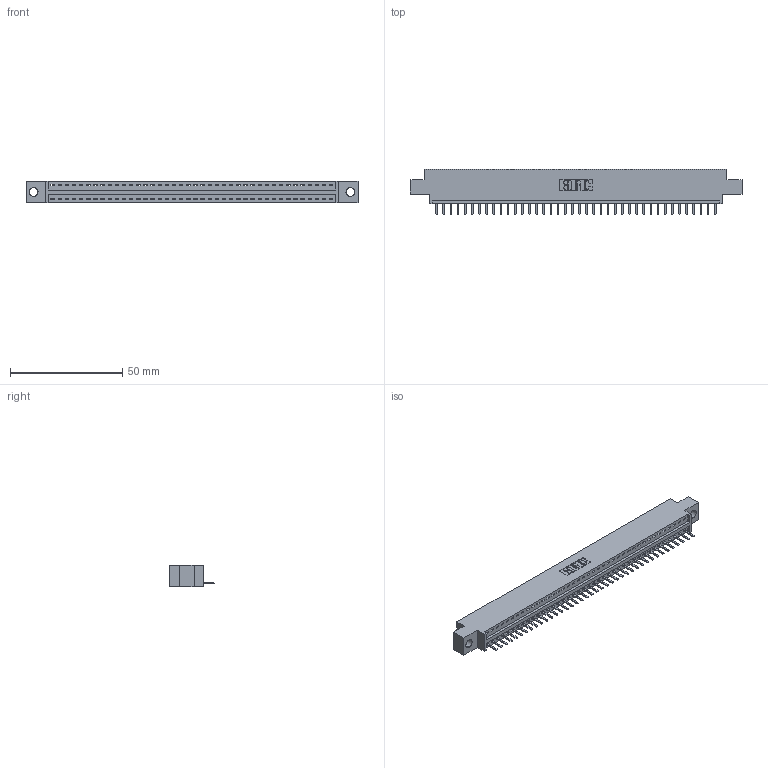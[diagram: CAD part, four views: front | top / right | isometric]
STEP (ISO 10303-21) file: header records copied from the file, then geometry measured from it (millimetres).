
FILE_DESCRIPTION (( 'STEP AP203' ), '1' );
FILE_NAME ('396-040-520-604.STEP', '2018-09-06T11:15:59', ( '' ), ( '' ), 'SwSTEP 2.0', 'SolidWorks 2016', '' );
FILE_SCHEMA (( 'CONFIG_CONTROL_DESIGN' ));
Length unit declared in the file: inch
Products named in the file (3): 396-040-520-604; 346 Part_0.170 Offset - 0.156 Dia-TH; 345-292-001_345-293-120
Assembly tree (41 placements, depth 2):
  396-040-520-604
    346 Part_0.170 Offset - 0.156 Dia-TH
    345-292-001_345-293-120  x40
Bounding box: 147.57 x 20.02 x 9.4 mm (x, y, z)
Volume: 13754.8 mm3; surface area: 16751.3 mm2
Topology: 41 solids, 41 shells, 2606 faces, 7701 edges, 5026 vertices
Faces by surface type: plane 1760, cylinder 846
Entity records: 25343 total; most frequent: CARTESIAN_POINT 4364, ORIENTED_EDGE 4326, DIRECTION 3839, EDGE_CURVE 2163, LINE 1867, VECTOR 1867, VERTEX_POINT 1438, AXIS2_PLACEMENT_3D 986
